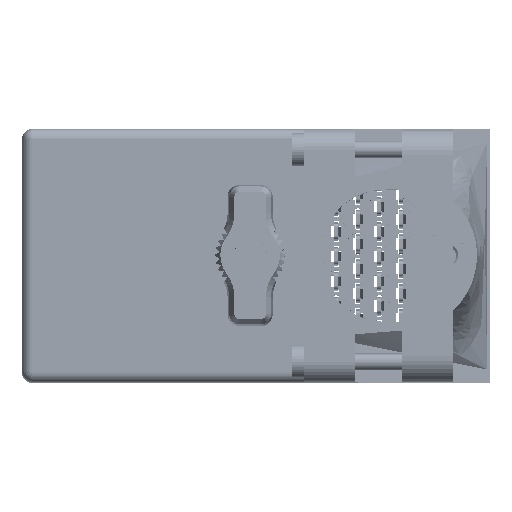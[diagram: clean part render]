
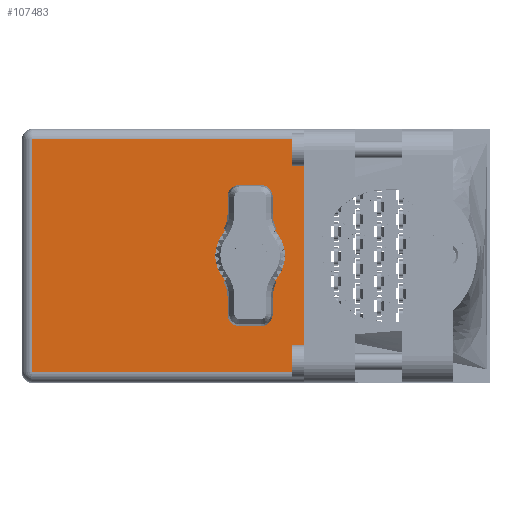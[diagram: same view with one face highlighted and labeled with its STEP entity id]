
A CAD part, top view. The second image highlights one B-rep face of the part: STEP entity #107483.
In plain terms, the highlighted face is planar.
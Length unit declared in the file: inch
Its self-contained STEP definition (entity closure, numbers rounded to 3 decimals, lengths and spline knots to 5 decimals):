
#474 = VERTEX_POINT ( 'NONE', #84397 ) ;
#9461 = ORIENTED_EDGE ( 'NONE', *, *, #86262, .T. ) ;
#14864 = FACE_OUTER_BOUND ( 'NONE', #22021, .T. ) ;
#15871 = CARTESIAN_POINT ( 'NONE',  ( 0., 2.03, -1.53 ) ) ;
#16741 = LINE ( 'NONE', #112292, #116116 ) ;
#17566 = CARTESIAN_POINT ( 'NONE',  ( 0., 2.03, -1.468 ) ) ;
#19708 = AXIS2_PLACEMENT_3D ( 'NONE', #57692, #111587, #39648 ) ;
#19981 = EDGE_CURVE ( 'NONE', #474, #105003, #104433, .T. ) ;
#22021 = EDGE_LOOP ( 'NONE', ( #9461, #83162, #48365, #98858 ) ) ;
#22116 = CARTESIAN_POINT ( 'NONE',  ( 1.705, 2.03, -0.062 ) ) ;
#24891 = FACE_BOUND ( 'NONE', #25271, .T. ) ;
#25156 = DIRECTION ( 'NONE',  ( 0., 1., 0. ) ) ;
#25271 = EDGE_LOOP ( 'NONE', ( #107356, #26553 ) ) ;
#26553 = ORIENTED_EDGE ( 'NONE', *, *, #56042, .F. ) ;
#28552 = EDGE_CURVE ( 'NONE', #58399, #65543, #37637, .T. ) ;
#29683 = VECTOR ( 'NONE', #108863, 39.37008 ) ;
#31822 = EDGE_CURVE ( 'NONE', #474, #65543, #16741, .T. ) ;
#32799 = CARTESIAN_POINT ( 'NONE',  ( 1.3775, 2.03, -0.765 ) ) ;
#34317 = CARTESIAN_POINT ( 'NONE',  ( 0.062, 2.03, -0.062 ) ) ;
#37637 = LINE ( 'NONE', #22116, #96618 ) ;
#39648 = DIRECTION ( 'NONE',  ( 0., 0., 1. ) ) ;
#43358 = VERTEX_POINT ( 'NONE', #116129 ) ;
#47043 = AXIS2_PLACEMENT_3D ( 'NONE', #15871, #25156, #62111 ) ;
#48365 = ORIENTED_EDGE ( 'NONE', *, *, #31822, .F. ) ;
#53263 = CIRCLE ( 'NONE', #54865, 0.1015 ) ;
#54865 = AXIS2_PLACEMENT_3D ( 'NONE', #32799, #97105, #97482 ) ;
#56042 = EDGE_CURVE ( 'NONE', #43358, #87566, #53263, .T. ) ;
#56051 = CIRCLE ( 'NONE', #19708, 0.1015 ) ;
#57208 = DIRECTION ( 'NONE',  ( 0., 0., 1. ) ) ;
#57692 = CARTESIAN_POINT ( 'NONE',  ( 1.3775, 2.03, -0.765 ) ) ;
#58399 = VERTEX_POINT ( 'NONE', #34317 ) ;
#62111 = DIRECTION ( 'NONE',  ( 0., 0., 1. ) ) ;
#64025 = DIRECTION ( 'NONE',  ( 0., 0., 1. ) ) ;
#65543 = VERTEX_POINT ( 'NONE', #92217 ) ;
#68412 = VECTOR ( 'NONE', #64025, 39.37008 ) ;
#68901 = CARTESIAN_POINT ( 'NONE',  ( 0.062, 2.03, -1.468 ) ) ;
#71312 = LINE ( 'NONE', #81306, #68412 ) ;
#76411 = DIRECTION ( 'NONE',  ( 1., 0., 0. ) ) ;
#78701 = CARTESIAN_POINT ( 'NONE',  ( 1.3775, 2.03, -0.6635 ) ) ;
#81306 = CARTESIAN_POINT ( 'NONE',  ( 0.062, 2.03, -1.53 ) ) ;
#83162 = ORIENTED_EDGE ( 'NONE', *, *, #28552, .T. ) ;
#84397 = CARTESIAN_POINT ( 'NONE',  ( 1.705, 2.03, -1.468 ) ) ;
#86262 = EDGE_CURVE ( 'NONE', #105003, #58399, #71312, .T. ) ;
#87566 = VERTEX_POINT ( 'NONE', #78701 ) ;
#92217 = CARTESIAN_POINT ( 'NONE',  ( 1.705, 2.03, -0.062 ) ) ;
#96618 = VECTOR ( 'NONE', #76411, 39.37008 ) ;
#97105 = DIRECTION ( 'NONE',  ( 0., 1., 0. ) ) ;
#97482 = DIRECTION ( 'NONE',  ( 0., 0., 1. ) ) ;
#98858 = ORIENTED_EDGE ( 'NONE', *, *, #19981, .T. ) ;
#102274 = EDGE_CURVE ( 'NONE', #87566, #43358, #56051, .T. ) ;
#104433 = LINE ( 'NONE', #17566, #29683 ) ;
#105003 = VERTEX_POINT ( 'NONE', #68901 ) ;
#107356 = ORIENTED_EDGE ( 'NONE', *, *, #102274, .F. ) ;
#107483 = ADVANCED_FACE ( 'NONE', ( #14864, #24891 ), #116816, .T. ) ;
#108863 = DIRECTION ( 'NONE',  ( -1., 0., 0. ) ) ;
#111587 = DIRECTION ( 'NONE',  ( 0., 1., 0. ) ) ;
#112292 = CARTESIAN_POINT ( 'NONE',  ( 1.705, 2.03, -1.53 ) ) ;
#116116 = VECTOR ( 'NONE', #57208, 39.37008 ) ;
#116129 = CARTESIAN_POINT ( 'NONE',  ( 1.3775, 2.03, -0.8665 ) ) ;
#116816 = PLANE ( 'NONE',  #47043 ) ;
